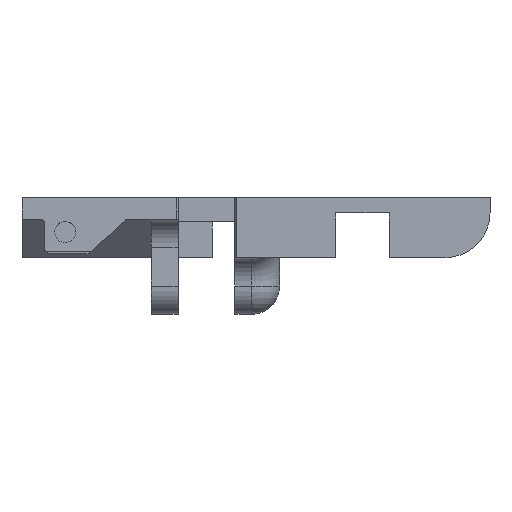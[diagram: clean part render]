
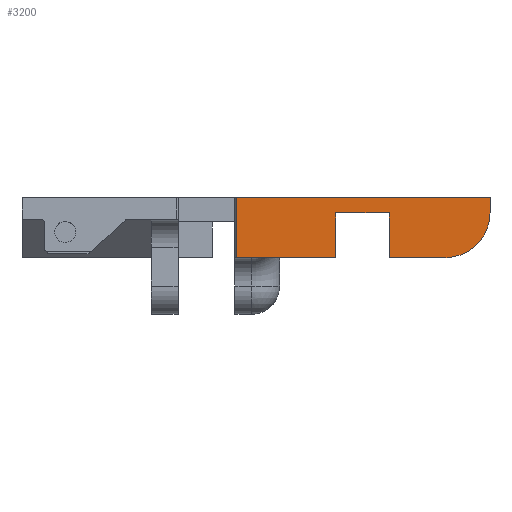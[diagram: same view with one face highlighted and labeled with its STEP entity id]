
A CAD part, left-side view. The second image highlights one B-rep face of the part: STEP entity #3200.
In plain terms, the highlighted planar face has unit normal (-1, 0, 0).
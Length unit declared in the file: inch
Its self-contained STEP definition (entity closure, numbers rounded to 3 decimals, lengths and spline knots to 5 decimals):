
#40 = VECTOR ( 'NONE', #3030, 39.37008 ) ;
#55 = CARTESIAN_POINT ( 'NONE',  ( -0.49053, -0.94414, -0.7732 ) ) ;
#159 = ORIENTED_EDGE ( 'NONE', *, *, #2001, .F. ) ;
#161 = CARTESIAN_POINT ( 'NONE',  ( -0.49053, -1.90672, -0.72597 ) ) ;
#182 = CARTESIAN_POINT ( 'NONE',  ( -0.49053, -2.04262, -0.61579 ) ) ;
#187 = LINE ( 'NONE', #536, #1039 ) ;
#199 = CARTESIAN_POINT ( 'NONE',  ( -0.49053, -1.61708, -0.73097 ) ) ;
#324 = DIRECTION ( 'NONE',  ( 0., 0., -1. ) ) ;
#383 = DIRECTION ( 'NONE',  ( 0., 0., -1. ) ) ;
#389 = EDGE_CURVE ( 'NONE', #1597, #4076, #3045, .T. ) ;
#467 = DIRECTION ( 'NONE',  ( 0., 1., 0. ) ) ;
#494 = CARTESIAN_POINT ( 'NONE',  ( -0.49053, -1.9254, -0.7207 ) ) ;
#511 = CARTESIAN_POINT ( 'NONE',  ( -0.49053, -2.05396, -0.58563 ) ) ;
#536 = CARTESIAN_POINT ( 'NONE',  ( -0.49053, -1.38086, -0.73097 ) ) ;
#617 = EDGE_LOOP ( 'NONE', ( #2193, #3593, #3504, #3219, #1409, #159, #1609, #3740, #730 ) ) ;
#645 = FACE_OUTER_BOUND ( 'NONE', #617, .T. ) ;
#705 = EDGE_CURVE ( 'NONE', #2415, #4076, #3634, .T. ) ;
#716 = CARTESIAN_POINT ( 'NONE',  ( -0.49053, -2.06046, 0. ) ) ;
#730 = ORIENTED_EDGE ( 'NONE', *, *, #389, .T. ) ;
#826 = CARTESIAN_POINT ( 'NONE',  ( -0.49053, -1.94956, -0.71115 ) ) ;
#837 = CARTESIAN_POINT ( 'NONE',  ( -0.49053, -2.06046, -0.54717 ) ) ;
#923 = LINE ( 'NONE', #1682, #40 ) ;
#924 = EDGE_CURVE ( 'NONE', #2625, #1733, #187, .T. ) ;
#976 = VECTOR ( 'NONE', #3456, 39.37008 ) ;
#1011 = VECTOR ( 'NONE', #383, 39.37008 ) ;
#1039 = VECTOR ( 'NONE', #2499, 39.37008 ) ;
#1062 = LINE ( 'NONE', #3442, #976 ) ;
#1079 = VECTOR ( 'NONE', #467, 39.37008 ) ;
#1092 = LINE ( 'NONE', #3779, #1868 ) ;
#1133 = EDGE_CURVE ( 'NONE', #2415, #2948, #1092, .T. ) ;
#1141 = CARTESIAN_POINT ( 'NONE',  ( -0.49053, -1.98248, -0.69093 ) ) ;
#1162 = CARTESIAN_POINT ( 'NONE',  ( -0.49053, -0.335, 0. ) ) ;
#1186 = VERTEX_POINT ( 'NONE', #2810 ) ;
#1348 = CARTESIAN_POINT ( 'NONE',  ( -0.49053, -1.61708, -0.53412 ) ) ;
#1353 = CARTESIAN_POINT ( 'NONE',  ( -0.49053, -1.38086, -0.53412 ) ) ;
#1409 = ORIENTED_EDGE ( 'NONE', *, *, #924, .F. ) ;
#1433 = CARTESIAN_POINT ( 'NONE',  ( -0.49053, -0.47716, -0.73097 ) ) ;
#1479 = CARTESIAN_POINT ( 'NONE',  ( -0.49053, -2.01106, -0.66454 ) ) ;
#1496 = DIRECTION ( 'NONE',  ( -1., 0., 0. ) ) ;
#1526 = CARTESIAN_POINT ( 'NONE',  ( -0.49053, -2.06046, -0.4665 ) ) ;
#1544 = CARTESIAN_POINT ( 'NONE',  ( -0.49053, -1.86189, -0.73097 ) ) ;
#1597 = VERTEX_POINT ( 'NONE', #1544 ) ;
#1609 = ORIENTED_EDGE ( 'NONE', *, *, #2664, .T. ) ;
#1682 = CARTESIAN_POINT ( 'NONE',  ( -0.49053, -1.61708, 0. ) ) ;
#1733 = VERTEX_POINT ( 'NONE', #1925 ) ;
#1759 = CARTESIAN_POINT ( 'NONE',  ( -0.49053, -0.47716, -0.73097 ) ) ;
#1785 = DIRECTION ( 'NONE',  ( 0., 1., 0. ) ) ;
#1796 = CARTESIAN_POINT ( 'NONE',  ( -0.49053, -2.03024, -0.63857 ) ) ;
#1868 = VECTOR ( 'NONE', #1785, 39.37008 ) ;
#1886 = LINE ( 'NONE', #55, #1011 ) ;
#1891 = LINE ( 'NONE', #1433, #2045 ) ;
#1925 = CARTESIAN_POINT ( 'NONE',  ( -0.49053, -1.38086, -0.73097 ) ) ;
#2001 = EDGE_CURVE ( 'NONE', #4195, #2625, #1062, .T. ) ;
#2045 = VECTOR ( 'NONE', #4080, 39.37008 ) ;
#2101 = CARTESIAN_POINT ( 'NONE',  ( -0.49053, -1.88778, -0.7297 ) ) ;
#2118 = CARTESIAN_POINT ( 'NONE',  ( -0.49053, -1.86189, -0.73097 ) ) ;
#2135 = CARTESIAN_POINT ( 'NONE',  ( -0.49053, -2.03983, -0.6216 ) ) ;
#2175 = LINE ( 'NONE', #1759, #1079 ) ;
#2193 = ORIENTED_EDGE ( 'NONE', *, *, #705, .F. ) ;
#2196 = CARTESIAN_POINT ( 'NONE',  ( -0.49053, -2.06046, -0.53412 ) ) ;
#2207 = EDGE_CURVE ( 'NONE', #1733, #1186, #1891, .T. ) ;
#2319 = VERTEX_POINT ( 'NONE', #199 ) ;
#2343 = CARTESIAN_POINT ( 'NONE',  ( -0.49053, -0.94414, -0.4665 ) ) ;
#2415 = VERTEX_POINT ( 'NONE', #1526 ) ;
#2458 = CARTESIAN_POINT ( 'NONE',  ( -0.49053, -1.91298, -0.72442 ) ) ;
#2473 = CARTESIAN_POINT ( 'NONE',  ( -0.49053, -2.05012, -0.59801 ) ) ;
#2499 = DIRECTION ( 'NONE',  ( 0., 0., -1. ) ) ;
#2625 = VERTEX_POINT ( 'NONE', #1353 ) ;
#2637 = EDGE_CURVE ( 'NONE', #2948, #1186, #1886, .T. ) ;
#2664 = EDGE_CURVE ( 'NONE', #4195, #2319, #923, .T. ) ;
#2746 = VECTOR ( 'NONE', #324, 39.37008 ) ;
#2787 = CARTESIAN_POINT ( 'NONE',  ( -0.49053, -1.93158, -0.71851 ) ) ;
#2804 = CARTESIAN_POINT ( 'NONE',  ( -0.49053, -2.05915, -0.56009 ) ) ;
#2810 = CARTESIAN_POINT ( 'NONE',  ( -0.49053, -0.94414, -0.73097 ) ) ;
#2948 = VERTEX_POINT ( 'NONE', #2343 ) ;
#3030 = DIRECTION ( 'NONE',  ( 0., 0., -1. ) ) ;
#3045 = B_SPLINE_CURVE_WITH_KNOTS ( 'NONE', 3,
 ( #2118, #4093, #2101, #161, #2458, #494, #2787, #826, #3126, #1141, #3458, #1479, #3791, #1796, #4130, #2135, #182, #2473, #511, #2804, #837, #2196 ),
 .UNSPECIFIED., .F., .F.,
 ( 4, 2, 2, 2, 2, 2, 2, 2, 2, 2, 4 ),
 ( 0., 0.00098, 0.00147, 0.00196, 0.00294, 0.00392, 0.0049, 0.00539, 0.00588, 0.00686, 0.00784 ),
 .UNSPECIFIED. ) ;
#3126 = CARTESIAN_POINT ( 'NONE',  ( -0.49053, -1.96093, -0.70513 ) ) ;
#3149 = PLANE ( 'NONE',  #3592 ) ;
#3200 = ADVANCED_FACE ( 'NONE', ( #645 ), #3149, .T. ) ;
#3219 = ORIENTED_EDGE ( 'NONE', *, *, #2207, .F. ) ;
#3442 = CARTESIAN_POINT ( 'NONE',  ( -0.49053, -1.38086, -0.53412 ) ) ;
#3456 = DIRECTION ( 'NONE',  ( 0., 1., 0. ) ) ;
#3458 = CARTESIAN_POINT ( 'NONE',  ( -0.49053, -1.9927, -0.68265 ) ) ;
#3504 = ORIENTED_EDGE ( 'NONE', *, *, #2637, .T. ) ;
#3592 = AXIS2_PLACEMENT_3D ( 'NONE', #1162, #1496, #3812 ) ;
#3593 = ORIENTED_EDGE ( 'NONE', *, *, #1133, .T. ) ;
#3634 = LINE ( 'NONE', #716, #2746 ) ;
#3740 = ORIENTED_EDGE ( 'NONE', *, *, #3785, .F. ) ;
#3779 = CARTESIAN_POINT ( 'NONE',  ( -0.49053, -0.335, -0.4665 ) ) ;
#3785 = EDGE_CURVE ( 'NONE', #1597, #2319, #2175, .T. ) ;
#3791 = CARTESIAN_POINT ( 'NONE',  ( -0.49053, -2.01931, -0.65466 ) ) ;
#3812 = DIRECTION ( 'NONE',  ( 0., -1., 0. ) ) ;
#3951 = CARTESIAN_POINT ( 'NONE',  ( -0.49053, -2.06046, -0.53412 ) ) ;
#4076 = VERTEX_POINT ( 'NONE', #3951 ) ;
#4080 = DIRECTION ( 'NONE',  ( 0., 1., 0. ) ) ;
#4093 = CARTESIAN_POINT ( 'NONE',  ( -0.49053, -1.87494, -0.73097 ) ) ;
#4130 = CARTESIAN_POINT ( 'NONE',  ( -0.49053, -2.03365, -0.63297 ) ) ;
#4195 = VERTEX_POINT ( 'NONE', #1348 ) ;
